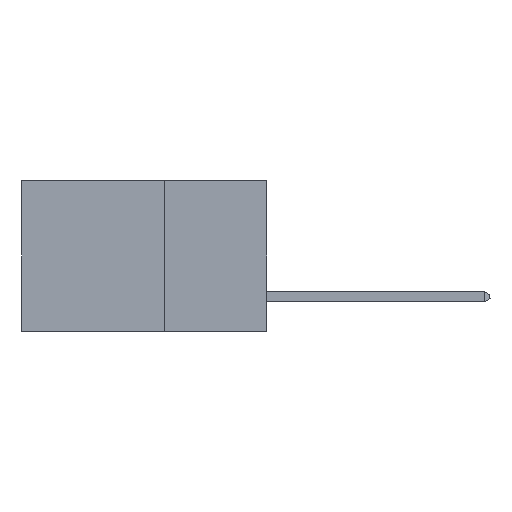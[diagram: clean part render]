
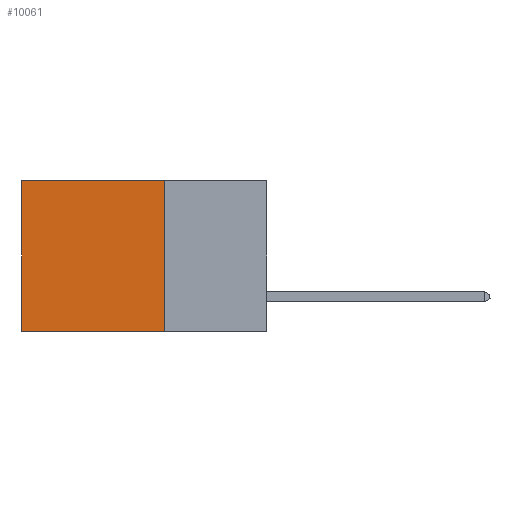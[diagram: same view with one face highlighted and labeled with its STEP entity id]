
A CAD part, left-side view. The second image highlights one B-rep face of the part: STEP entity #10061.
In plain terms, the highlighted planar face has unit normal (-1, 0, 0).
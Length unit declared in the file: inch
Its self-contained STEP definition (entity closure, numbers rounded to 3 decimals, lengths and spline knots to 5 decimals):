
#383 = DIRECTION ( 'NONE',  ( 0., 0., -1. ) ) ;
#422 = CARTESIAN_POINT ( 'NONE',  ( 0.2875, 0.25, -0.37 ) ) ;
#439 = PLANE ( 'NONE',  #13214 ) ;
#778 = EDGE_LOOP ( 'NONE', ( #18189, #1617, #13972, #15472 ) ) ;
#1617 = ORIENTED_EDGE ( 'NONE', *, *, #3514, .F. ) ;
#1946 = CARTESIAN_POINT ( 'NONE',  ( 0.2875, 0.25, -0.37 ) ) ;
#3514 = EDGE_CURVE ( 'NONE', #15066, #5339, #7714, .T. ) ;
#3755 = DIRECTION ( 'NONE',  ( 0., 1., 0. ) ) ;
#4208 = CARTESIAN_POINT ( 'NONE',  ( 0.2875, 0.25, 0. ) ) ;
#4336 = FACE_OUTER_BOUND ( 'NONE', #778, .T. ) ;
#5339 = VERTEX_POINT ( 'NONE', #15272 ) ;
#5725 = LINE ( 'NONE', #16857, #12220 ) ;
#6071 = VERTEX_POINT ( 'NONE', #6468 ) ;
#6468 = CARTESIAN_POINT ( 'NONE',  ( 0.2875, 0.25, 0. ) ) ;
#6558 = EDGE_CURVE ( 'NONE', #6071, #15066, #15117, .T. ) ;
#7714 = LINE ( 'NONE', #1946, #19044 ) ;
#7854 = VECTOR ( 'NONE', #3755, 39.37008 ) ;
#9490 = CARTESIAN_POINT ( 'NONE',  ( 0.2875, 0.25, 0. ) ) ;
#9545 = EDGE_CURVE ( 'NONE', #14709, #5339, #5725, .T. ) ;
#9590 = DIRECTION ( 'NONE',  ( 0., 0., -1. ) ) ;
#9937 = LINE ( 'NONE', #9490, #7854 ) ;
#10061 = ADVANCED_FACE ( 'NONE', ( #4336 ), #439, .F. ) ;
#10828 = DIRECTION ( 'NONE',  ( 1., 0., 0. ) ) ;
#12220 = VECTOR ( 'NONE', #383, 39.37008 ) ;
#12235 = CARTESIAN_POINT ( 'NONE',  ( 0.2875, 0.25, 0. ) ) ;
#13133 = EDGE_CURVE ( 'NONE', #6071, #14709, #9937, .T. ) ;
#13214 = AXIS2_PLACEMENT_3D ( 'NONE', #12235, #10828, #9590 ) ;
#13972 = ORIENTED_EDGE ( 'NONE', *, *, #6558, .F. ) ;
#14208 = CARTESIAN_POINT ( 'NONE',  ( 0.2875, 0.6, 0. ) ) ;
#14709 = VERTEX_POINT ( 'NONE', #14208 ) ;
#15066 = VERTEX_POINT ( 'NONE', #422 ) ;
#15117 = LINE ( 'NONE', #4208, #17673 ) ;
#15272 = CARTESIAN_POINT ( 'NONE',  ( 0.2875, 0.6, -0.37 ) ) ;
#15472 = ORIENTED_EDGE ( 'NONE', *, *, #13133, .T. ) ;
#15904 = DIRECTION ( 'NONE',  ( 0., 0., -1. ) ) ;
#16857 = CARTESIAN_POINT ( 'NONE',  ( 0.2875, 0.6, 0. ) ) ;
#17673 = VECTOR ( 'NONE', #15904, 39.37008 ) ;
#18189 = ORIENTED_EDGE ( 'NONE', *, *, #9545, .T. ) ;
#18265 = DIRECTION ( 'NONE',  ( 0., 1., 0. ) ) ;
#19044 = VECTOR ( 'NONE', #18265, 39.37008 ) ;
